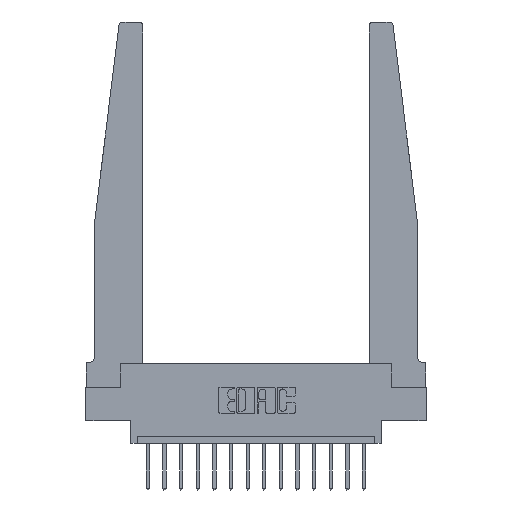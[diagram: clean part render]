
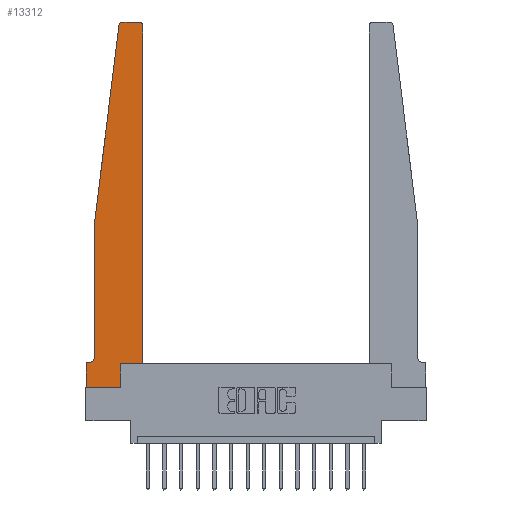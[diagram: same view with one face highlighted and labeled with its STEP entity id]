
A CAD part, top view. The second image highlights one B-rep face of the part: STEP entity #13312.
In plain terms, the highlighted planar face has unit normal (0, 0, 1).
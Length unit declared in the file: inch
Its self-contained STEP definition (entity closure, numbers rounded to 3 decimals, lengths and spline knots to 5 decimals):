
#89 = CARTESIAN_POINT ( 'NONE',  ( 0., 0.1875, 0.37 ) ) ;
#187 = EDGE_CURVE ( 'NONE', #11477, #17657, #7416, .T. ) ;
#237 = VERTEX_POINT ( 'NONE', #11483 ) ;
#330 = DIRECTION ( 'NONE',  ( -1., 0., 0. ) ) ;
#456 = CARTESIAN_POINT ( 'NONE',  ( 0.2605, 0., 0.37 ) ) ;
#861 = DIRECTION ( 'NONE',  ( -1., 0., 0. ) ) ;
#1274 = LINE ( 'NONE', #17661, #7998 ) ;
#1404 = VECTOR ( 'NONE', #330, 39.37008 ) ;
#1477 = CARTESIAN_POINT ( 'NONE',  ( 0.065, 1.25, 0.37 ) ) ;
#1589 = EDGE_CURVE ( 'NONE', #14846, #3812, #17505, .T. ) ;
#1942 = DIRECTION ( 'NONE',  ( 0., -1., 0. ) ) ;
#2160 = EDGE_CURVE ( 'NONE', #13769, #2516, #4040, .T. ) ;
#2516 = VERTEX_POINT ( 'NONE', #13340 ) ;
#2559 = CARTESIAN_POINT ( 'NONE',  ( 0.2605, 0.18, 0.37 ) ) ;
#2892 = DIRECTION ( 'NONE',  ( 0., 0., 1. ) ) ;
#2918 = CARTESIAN_POINT ( 'NONE',  ( 0.24675, 2.72367, 0.37 ) ) ;
#2978 = CARTESIAN_POINT ( 'NONE',  ( 0., 0.1875, 0.37 ) ) ;
#3524 = VECTOR ( 'NONE', #8919, 39.37008 ) ;
#3678 = VECTOR ( 'NONE', #861, 39.37008 ) ;
#3694 = EDGE_CURVE ( 'NONE', #17657, #12833, #13618, .T. ) ;
#3767 = EDGE_CURVE ( 'NONE', #15835, #8681, #6136, .T. ) ;
#3805 = CARTESIAN_POINT ( 'NONE',  ( 0.065, 1.25, 0.37 ) ) ;
#3812 = VERTEX_POINT ( 'NONE', #2918 ) ;
#3867 = LINE ( 'NONE', #9634, #5138 ) ;
#3888 = AXIS2_PLACEMENT_3D ( 'NONE', #15807, #6348, #4900 ) ;
#4006 = CARTESIAN_POINT ( 'NONE',  ( 0.425, 0.18, 0.37 ) ) ;
#4040 = CIRCLE ( 'NONE', #14119, 0.03 ) ;
#4584 = FACE_OUTER_BOUND ( 'NONE', #17723, .T. ) ;
#4841 = ORIENTED_EDGE ( 'NONE', *, *, #12184, .T. ) ;
#4900 = DIRECTION ( 'NONE',  ( -1., 0., 0. ) ) ;
#5004 = ORIENTED_EDGE ( 'NONE', *, *, #2160, .T. ) ;
#5048 = CARTESIAN_POINT ( 'NONE',  ( 0.425, 2.72, 0.37 ) ) ;
#5138 = VECTOR ( 'NONE', #6574, 39.37008 ) ;
#5323 = DIRECTION ( 'NONE',  ( -0.122, -0.992, 0. ) ) ;
#5933 = LINE ( 'NONE', #11423, #9126 ) ;
#5956 = EDGE_CURVE ( 'NONE', #237, #11477, #12666, .T. ) ;
#6092 = CARTESIAN_POINT ( 'NONE',  ( 0.065, 0.2375, 0.37 ) ) ;
#6136 = LINE ( 'NONE', #1477, #3524 ) ;
#6348 = DIRECTION ( 'NONE',  ( 0., 0., -1. ) ) ;
#6442 = LINE ( 'NONE', #13365, #3678 ) ;
#6574 = DIRECTION ( 'NONE',  ( 0., 1., 0. ) ) ;
#6708 = EDGE_CURVE ( 'NONE', #17660, #7273, #14817, .T. ) ;
#6843 = ORIENTED_EDGE ( 'NONE', *, *, #3694, .T. ) ;
#7273 = VERTEX_POINT ( 'NONE', #4006 ) ;
#7416 = LINE ( 'NONE', #17146, #13303 ) ;
#7543 = DIRECTION ( 'NONE',  ( 1., 0., 0. ) ) ;
#7672 = CARTESIAN_POINT ( 'NONE',  ( 0.27653, 2.72, 0.37 ) ) ;
#7959 = ORIENTED_EDGE ( 'NONE', *, *, #187, .T. ) ;
#7998 = VECTOR ( 'NONE', #5323, 39.37008 ) ;
#8094 = VECTOR ( 'NONE', #14694, 39.37008 ) ;
#8349 = ORIENTED_EDGE ( 'NONE', *, *, #11590, .T. ) ;
#8681 = VERTEX_POINT ( 'NONE', #6092 ) ;
#8822 = EDGE_CURVE ( 'NONE', #8681, #237, #14792, .T. ) ;
#8919 = DIRECTION ( 'NONE',  ( 0., -1., 0. ) ) ;
#9126 = VECTOR ( 'NONE', #16914, 39.37008 ) ;
#9387 = ORIENTED_EDGE ( 'NONE', *, *, #5956, .T. ) ;
#9464 = CARTESIAN_POINT ( 'NONE',  ( 0.395, 2.72, 0.37 ) ) ;
#9634 = CARTESIAN_POINT ( 'NONE',  ( 0.425, 0.18, 0.37 ) ) ;
#9985 = ORIENTED_EDGE ( 'NONE', *, *, #3767, .T. ) ;
#10000 = PLANE ( 'NONE',  #14912 ) ;
#10445 = VECTOR ( 'NONE', #7543, 39.37008 ) ;
#11026 = CARTESIAN_POINT ( 'NONE',  ( 0., 0., 0.37 ) ) ;
#11242 = CARTESIAN_POINT ( 'NONE',  ( 0.065, 0.1875, 0.37 ) ) ;
#11423 = CARTESIAN_POINT ( 'NONE',  ( 0.2605, 0.18, 0.37 ) ) ;
#11477 = VERTEX_POINT ( 'NONE', #89 ) ;
#11483 = CARTESIAN_POINT ( 'NONE',  ( 0.015, 0.1875, 0.37 ) ) ;
#11590 = EDGE_CURVE ( 'NONE', #12833, #17660, #5933, .T. ) ;
#11916 = DIRECTION ( 'NONE',  ( 0., 0., 1. ) ) ;
#12184 = EDGE_CURVE ( 'NONE', #2516, #14846, #6442, .T. ) ;
#12246 = DIRECTION ( 'NONE',  ( 1., 0., 0. ) ) ;
#12656 = EDGE_CURVE ( 'NONE', #3812, #15835, #1274, .T. ) ;
#12666 = LINE ( 'NONE', #11242, #1404 ) ;
#12833 = VERTEX_POINT ( 'NONE', #456 ) ;
#12896 = ORIENTED_EDGE ( 'NONE', *, *, #13104, .T. ) ;
#13061 = ORIENTED_EDGE ( 'NONE', *, *, #6708, .T. ) ;
#13104 = EDGE_CURVE ( 'NONE', #7273, #13769, #3867, .T. ) ;
#13222 = CARTESIAN_POINT ( 'NONE',  ( 0.425, 0.18, 0.37 ) ) ;
#13303 = VECTOR ( 'NONE', #1942, 39.37008 ) ;
#13312 = ADVANCED_FACE ( 'NONE', ( #4584 ), #10000, .T. ) ;
#13340 = CARTESIAN_POINT ( 'NONE',  ( 0.395, 2.75, 0.37 ) ) ;
#13365 = CARTESIAN_POINT ( 'NONE',  ( 0.25, 2.75, 0.37 ) ) ;
#13451 = CARTESIAN_POINT ( 'NONE',  ( 0., 0., 0.37 ) ) ;
#13618 = LINE ( 'NONE', #11026, #8094 ) ;
#13689 = CARTESIAN_POINT ( 'NONE',  ( 0.27653, 2.75, 0.37 ) ) ;
#13769 = VERTEX_POINT ( 'NONE', #5048 ) ;
#14021 = ORIENTED_EDGE ( 'NONE', *, *, #8822, .T. ) ;
#14119 = AXIS2_PLACEMENT_3D ( 'NONE', #9464, #2892, #12246 ) ;
#14694 = DIRECTION ( 'NONE',  ( 1., 0., 0. ) ) ;
#14792 = CIRCLE ( 'NONE', #3888, 0.05 ) ;
#14817 = LINE ( 'NONE', #13222, #10445 ) ;
#14846 = VERTEX_POINT ( 'NONE', #13689 ) ;
#14912 = AXIS2_PLACEMENT_3D ( 'NONE', #2978, #16831, #16570 ) ;
#14977 = ORIENTED_EDGE ( 'NONE', *, *, #12656, .T. ) ;
#15807 = CARTESIAN_POINT ( 'NONE',  ( 0.015, 0.2375, 0.37 ) ) ;
#15835 = VERTEX_POINT ( 'NONE', #3805 ) ;
#16075 = AXIS2_PLACEMENT_3D ( 'NONE', #7672, #11916, #17322 ) ;
#16570 = DIRECTION ( 'NONE',  ( 1., 0., 0. ) ) ;
#16831 = DIRECTION ( 'NONE',  ( 0., 0., 1. ) ) ;
#16914 = DIRECTION ( 'NONE',  ( 0., 1., 0. ) ) ;
#17146 = CARTESIAN_POINT ( 'NONE',  ( 0., 0., 0.37 ) ) ;
#17322 = DIRECTION ( 'NONE',  ( 1., 0., 0. ) ) ;
#17421 = ORIENTED_EDGE ( 'NONE', *, *, #1589, .T. ) ;
#17505 = CIRCLE ( 'NONE', #16075, 0.03 ) ;
#17657 = VERTEX_POINT ( 'NONE', #13451 ) ;
#17660 = VERTEX_POINT ( 'NONE', #2559 ) ;
#17661 = CARTESIAN_POINT ( 'NONE',  ( 0.065, 1.25, 0.37 ) ) ;
#17723 = EDGE_LOOP ( 'NONE', ( #4841, #17421, #14977, #9985, #14021, #9387, #7959, #6843, #8349, #13061, #12896, #5004 ) ) ;
